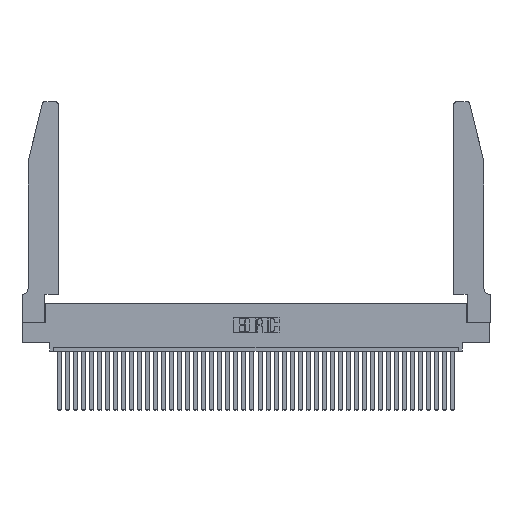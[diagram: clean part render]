
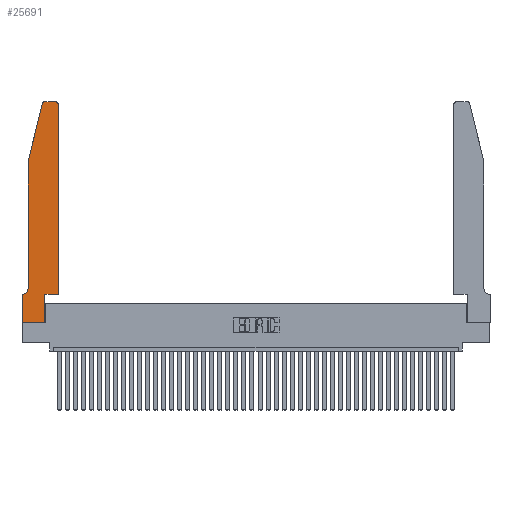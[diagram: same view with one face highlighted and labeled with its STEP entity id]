
A CAD part, top view. The second image highlights one B-rep face of the part: STEP entity #25691.
In plain terms, the highlighted planar face has unit normal (0, 0, 1).
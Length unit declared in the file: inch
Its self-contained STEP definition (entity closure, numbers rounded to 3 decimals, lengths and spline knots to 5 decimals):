
#119 = ORIENTED_EDGE ( 'NONE', *, *, #35320, .T. ) ;
#631 = VERTEX_POINT ( 'NONE', #37694 ) ;
#890 = DIRECTION ( 'NONE',  ( 0., 0., 1. ) ) ;
#2127 = LINE ( 'NONE', #19463, #5122 ) ;
#2307 = DIRECTION ( 'NONE',  ( 0., 0., 1. ) ) ;
#2693 = VERTEX_POINT ( 'NONE', #29211 ) ;
#2749 = ORIENTED_EDGE ( 'NONE', *, *, #28760, .T. ) ;
#2900 = CARTESIAN_POINT ( 'NONE',  ( 0.2865, 0.35, 0.37 ) ) ;
#2975 = CIRCLE ( 'NONE', #34049, 0.03 ) ;
#3052 = VERTEX_POINT ( 'NONE', #28254 ) ;
#3553 = ORIENTED_EDGE ( 'NONE', *, *, #22244, .T. ) ;
#3615 = DIRECTION ( 'NONE',  ( 1., 0., 0. ) ) ;
#3944 = DIRECTION ( 'NONE',  ( 1., 0., 0. ) ) ;
#5122 = VECTOR ( 'NONE', #3615, 39.37008 ) ;
#5413 = EDGE_CURVE ( 'NONE', #12736, #30597, #2975, .T. ) ;
#5737 = VERTEX_POINT ( 'NONE', #13859 ) ;
#6592 = LINE ( 'NONE', #12303, #38943 ) ;
#7401 = DIRECTION ( 'NONE',  ( 1., 0., 0. ) ) ;
#7749 = VECTOR ( 'NONE', #16334, 39.37008 ) ;
#8129 = CARTESIAN_POINT ( 'NONE',  ( 0.4205, 2.72, 0.37 ) ) ;
#8462 = CARTESIAN_POINT ( 'NONE',  ( 0.284, 2.75, 0.37 ) ) ;
#8551 = DIRECTION ( 'NONE',  ( -0.239, -0.971, 0. ) ) ;
#8735 = CARTESIAN_POINT ( 'NONE',  ( 0.0755, 0.35, 0.37 ) ) ;
#9223 = LINE ( 'NONE', #8735, #15652 ) ;
#9788 = CARTESIAN_POINT ( 'NONE',  ( 0.4505, 2.72, 0.37 ) ) ;
#10134 = CARTESIAN_POINT ( 'NONE',  ( 0., 0.35, 0.37 ) ) ;
#10579 = CARTESIAN_POINT ( 'NONE',  ( 0.0055, 0.42, 0.37 ) ) ;
#10658 = CARTESIAN_POINT ( 'NONE',  ( 0.4505, 0.35, 0.37 ) ) ;
#10700 = EDGE_CURVE ( 'NONE', #12660, #12736, #26348, .T. ) ;
#10858 = DIRECTION ( 'NONE',  ( -1., 0., 0. ) ) ;
#11066 = CARTESIAN_POINT ( 'NONE',  ( 0.0755, 2., 0.37 ) ) ;
#12252 = ORIENTED_EDGE ( 'NONE', *, *, #14575, .T. ) ;
#12303 = CARTESIAN_POINT ( 'NONE',  ( 0., 0., 0.37 ) ) ;
#12660 = VERTEX_POINT ( 'NONE', #30771 ) ;
#12707 = AXIS2_PLACEMENT_3D ( 'NONE', #10579, #19980, #10858 ) ;
#12736 = VERTEX_POINT ( 'NONE', #9788 ) ;
#12937 = ORIENTED_EDGE ( 'NONE', *, *, #32757, .T. ) ;
#12993 = FACE_OUTER_BOUND ( 'NONE', #20506, .T. ) ;
#13422 = CARTESIAN_POINT ( 'NONE',  ( 0.0755, 2., 0.37 ) ) ;
#13530 = LINE ( 'NONE', #40642, #17531 ) ;
#13746 = DIRECTION ( 'NONE',  ( 1., 0., 0. ) ) ;
#13859 = CARTESIAN_POINT ( 'NONE',  ( 0.0755, 0.42, 0.37 ) ) ;
#14575 = EDGE_CURVE ( 'NONE', #35619, #21890, #31483, .T. ) ;
#15652 = VECTOR ( 'NONE', #30532, 39.37008 ) ;
#16334 = DIRECTION ( 'NONE',  ( 0., -1., 0. ) ) ;
#17047 = ORIENTED_EDGE ( 'NONE', *, *, #27175, .T. ) ;
#17531 = VECTOR ( 'NONE', #18456, 39.37008 ) ;
#18456 = DIRECTION ( 'NONE',  ( -1., 0., 0. ) ) ;
#19196 = DIRECTION ( 'NONE',  ( 0., 0., 1. ) ) ;
#19463 = CARTESIAN_POINT ( 'NONE',  ( 0.4505, 0.35, 0.37 ) ) ;
#19910 = DIRECTION ( 'NONE',  ( 0., 1., 0. ) ) ;
#19920 = CARTESIAN_POINT ( 'NONE',  ( 0.4205, 2.75, 0.37 ) ) ;
#19956 = PLANE ( 'NONE',  #23075 ) ;
#19972 = VERTEX_POINT ( 'NONE', #8462 ) ;
#19980 = DIRECTION ( 'NONE',  ( 0., 0., -1. ) ) ;
#20119 = LINE ( 'NONE', #13422, #7749 ) ;
#20506 = EDGE_LOOP ( 'NONE', ( #39352, #17047, #3553, #2749, #12937, #27662, #31530, #12252, #119, #31067, #21279, #40316 ) ) ;
#21279 = ORIENTED_EDGE ( 'NONE', *, *, #10700, .T. ) ;
#21836 = EDGE_CURVE ( 'NONE', #631, #35619, #6592, .T. ) ;
#21890 = VERTEX_POINT ( 'NONE', #29493 ) ;
#22244 = EDGE_CURVE ( 'NONE', #3052, #34054, #36937, .T. ) ;
#22415 = VECTOR ( 'NONE', #19910, 39.37008 ) ;
#23075 = AXIS2_PLACEMENT_3D ( 'NONE', #10134, #890, #13746 ) ;
#24521 = VECTOR ( 'NONE', #3944, 39.37008 ) ;
#25304 = CIRCLE ( 'NONE', #30398, 0.03 ) ;
#25691 = ADVANCED_FACE ( 'NONE', ( #12993 ), #19956, .T. ) ;
#26348 = LINE ( 'NONE', #10658, #22415 ) ;
#27175 = EDGE_CURVE ( 'NONE', #19972, #3052, #25304, .T. ) ;
#27662 = ORIENTED_EDGE ( 'NONE', *, *, #39870, .T. ) ;
#28254 = CARTESIAN_POINT ( 'NONE',  ( 0.25487, 2.72718, 0.37 ) ) ;
#28337 = DIRECTION ( 'NONE',  ( 0., 1., 0. ) ) ;
#28760 = EDGE_CURVE ( 'NONE', #34054, #5737, #20119, .T. ) ;
#29211 = CARTESIAN_POINT ( 'NONE',  ( 0.2865, 0.35, 0.37 ) ) ;
#29493 = CARTESIAN_POINT ( 'NONE',  ( 0.2865, 0., 0.37 ) ) ;
#30398 = AXIS2_PLACEMENT_3D ( 'NONE', #37252, #2307, #30971 ) ;
#30532 = DIRECTION ( 'NONE',  ( -1., 0., 0. ) ) ;
#30597 = VERTEX_POINT ( 'NONE', #19920 ) ;
#30771 = CARTESIAN_POINT ( 'NONE',  ( 0.4505, 0.35, 0.37 ) ) ;
#30971 = DIRECTION ( 'NONE',  ( 1., 0., 0. ) ) ;
#31067 = ORIENTED_EDGE ( 'NONE', *, *, #40350, .T. ) ;
#31465 = VECTOR ( 'NONE', #8551, 39.37008 ) ;
#31483 = LINE ( 'NONE', #35548, #24521 ) ;
#31530 = ORIENTED_EDGE ( 'NONE', *, *, #21836, .T. ) ;
#31863 = EDGE_CURVE ( 'NONE', #30597, #19972, #13530, .T. ) ;
#31865 = CIRCLE ( 'NONE', #12707, 0.07 ) ;
#32216 = VERTEX_POINT ( 'NONE', #39852 ) ;
#32574 = CARTESIAN_POINT ( 'NONE',  ( 0., 0., 0.37 ) ) ;
#32757 = EDGE_CURVE ( 'NONE', #5737, #32216, #31865, .T. ) ;
#34049 = AXIS2_PLACEMENT_3D ( 'NONE', #8129, #19196, #7401 ) ;
#34054 = VERTEX_POINT ( 'NONE', #11066 ) ;
#35320 = EDGE_CURVE ( 'NONE', #21890, #2693, #39682, .T. ) ;
#35548 = CARTESIAN_POINT ( 'NONE',  ( 0., 0., 0.37 ) ) ;
#35619 = VERTEX_POINT ( 'NONE', #32574 ) ;
#36937 = LINE ( 'NONE', #37329, #31465 ) ;
#37252 = CARTESIAN_POINT ( 'NONE',  ( 0.284, 2.72, 0.37 ) ) ;
#37329 = CARTESIAN_POINT ( 'NONE',  ( 0.0755, 2., 0.37 ) ) ;
#37694 = CARTESIAN_POINT ( 'NONE',  ( 0., 0.35, 0.37 ) ) ;
#38640 = VECTOR ( 'NONE', #28337, 39.37008 ) ;
#38943 = VECTOR ( 'NONE', #40698, 39.37008 ) ;
#39352 = ORIENTED_EDGE ( 'NONE', *, *, #31863, .T. ) ;
#39682 = LINE ( 'NONE', #2900, #38640 ) ;
#39852 = CARTESIAN_POINT ( 'NONE',  ( 0.0055, 0.35, 0.37 ) ) ;
#39870 = EDGE_CURVE ( 'NONE', #32216, #631, #9223, .T. ) ;
#40316 = ORIENTED_EDGE ( 'NONE', *, *, #5413, .T. ) ;
#40350 = EDGE_CURVE ( 'NONE', #2693, #12660, #2127, .T. ) ;
#40642 = CARTESIAN_POINT ( 'NONE',  ( 0.2605, 2.75, 0.37 ) ) ;
#40698 = DIRECTION ( 'NONE',  ( 0., -1., 0. ) ) ;
